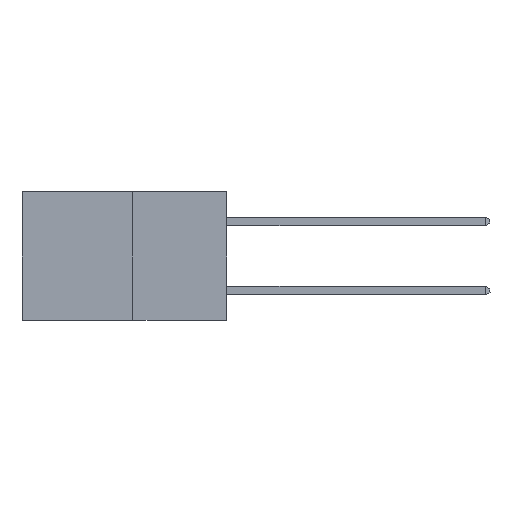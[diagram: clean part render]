
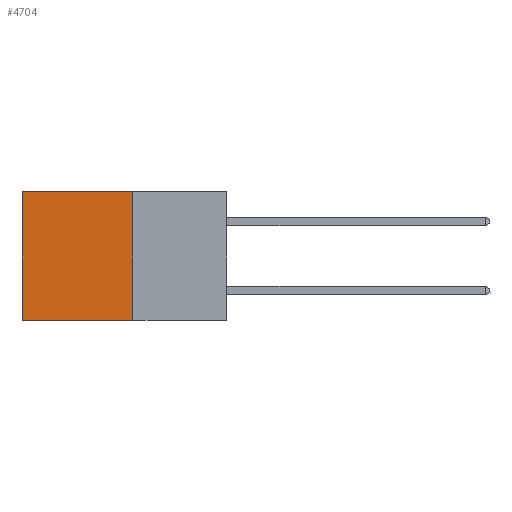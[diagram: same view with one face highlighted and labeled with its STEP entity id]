
A CAD part, left-side view. The second image highlights one B-rep face of the part: STEP entity #4704.
In plain terms, the highlighted planar face has unit normal (-1, 0, 0).
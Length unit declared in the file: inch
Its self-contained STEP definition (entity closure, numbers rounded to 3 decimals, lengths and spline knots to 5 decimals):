
#1678 = VERTEX_POINT ( 'NONE', #26748 ) ;
#2631 = EDGE_CURVE ( 'NONE', #22548, #1678, #23199, .T. ) ;
#3704 = DIRECTION ( 'NONE',  ( 0., 0., -1. ) ) ;
#3802 = CARTESIAN_POINT ( 'NONE',  ( 0.277, 0.27, -0.37 ) ) ;
#4434 = ORIENTED_EDGE ( 'NONE', *, *, #2631, .T. ) ;
#4704 = ADVANCED_FACE ( 'NONE', ( #21677 ), #21935, .F. ) ;
#5128 = VECTOR ( 'NONE', #18274, 39.37008 ) ;
#5719 = EDGE_CURVE ( 'NONE', #22548, #26387, #9043, .T. ) ;
#6438 = EDGE_LOOP ( 'NONE', ( #12202, #22569, #18820, #4434 ) ) ;
#7886 = CARTESIAN_POINT ( 'NONE',  ( 0.277, 0.59, -0.37 ) ) ;
#8857 = AXIS2_PLACEMENT_3D ( 'NONE', #21930, #21831, #21775 ) ;
#9043 = LINE ( 'NONE', #3802, #20919 ) ;
#10293 = DIRECTION ( 'NONE',  ( 0., 0., -1. ) ) ;
#12202 = ORIENTED_EDGE ( 'NONE', *, *, #19273, .T. ) ;
#12315 = CARTESIAN_POINT ( 'NONE',  ( 0.277, 0.27, -0.37 ) ) ;
#14274 = VECTOR ( 'NONE', #10293, 39.37008 ) ;
#14385 = VECTOR ( 'NONE', #18859, 39.37008 ) ;
#16126 = CARTESIAN_POINT ( 'NONE',  ( 0.277, 0.27, 0. ) ) ;
#16482 = CARTESIAN_POINT ( 'NONE',  ( 0.277, 0.27, -0.37 ) ) ;
#16856 = CARTESIAN_POINT ( 'NONE',  ( 0.277, 0.59, -0.37 ) ) ;
#18274 = DIRECTION ( 'NONE',  ( 0., 1., 0. ) ) ;
#18820 = ORIENTED_EDGE ( 'NONE', *, *, #5719, .F. ) ;
#18859 = DIRECTION ( 'NONE',  ( 0., 1., 0. ) ) ;
#19273 = EDGE_CURVE ( 'NONE', #1678, #20110, #20566, .T. ) ;
#19732 = CARTESIAN_POINT ( 'NONE',  ( 0.277, 0.27, 0. ) ) ;
#20110 = VERTEX_POINT ( 'NONE', #16856 ) ;
#20566 = LINE ( 'NONE', #7886, #14274 ) ;
#20919 = VECTOR ( 'NONE', #3704, 39.37008 ) ;
#21677 = FACE_OUTER_BOUND ( 'NONE', #6438, .T. ) ;
#21775 = DIRECTION ( 'NONE',  ( 0., 0., -1. ) ) ;
#21831 = DIRECTION ( 'NONE',  ( 1., 0., 0. ) ) ;
#21930 = CARTESIAN_POINT ( 'NONE',  ( 0.277, 0.27, -0.37 ) ) ;
#21935 = PLANE ( 'NONE',  #8857 ) ;
#22548 = VERTEX_POINT ( 'NONE', #16126 ) ;
#22569 = ORIENTED_EDGE ( 'NONE', *, *, #27656, .F. ) ;
#23199 = LINE ( 'NONE', #19732, #5128 ) ;
#26387 = VERTEX_POINT ( 'NONE', #12315 ) ;
#26748 = CARTESIAN_POINT ( 'NONE',  ( 0.277, 0.59, 0. ) ) ;
#26831 = LINE ( 'NONE', #16482, #14385 ) ;
#27656 = EDGE_CURVE ( 'NONE', #26387, #20110, #26831, .T. ) ;
